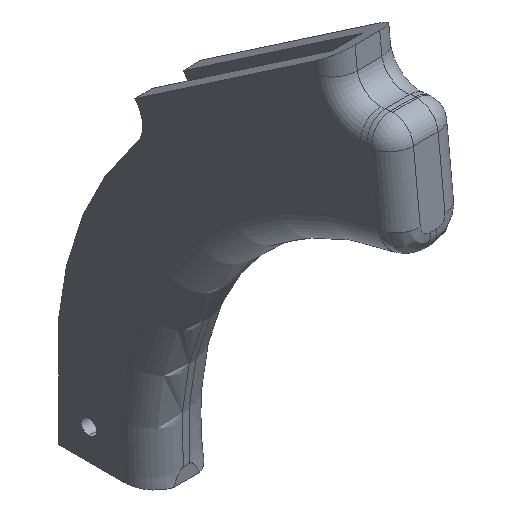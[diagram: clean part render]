
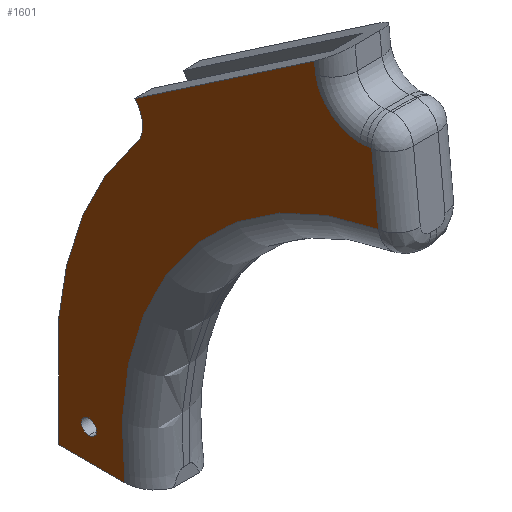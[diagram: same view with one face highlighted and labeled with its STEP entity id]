
A CAD part, isometric view. The second image highlights one B-rep face of the part: STEP entity #1601.
In plain terms, the highlighted planar face has unit normal (-1, 0, 0).
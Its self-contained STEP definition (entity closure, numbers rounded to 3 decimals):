
#111 = ORIENTED_EDGE ( 'NONE', *, *, #1581, .F. ) ;
#112 = ORIENTED_EDGE ( 'NONE', *, *, #1582, .T. ) ;
#113 = ORIENTED_EDGE ( 'NONE', *, *, #1477, .F. ) ;
#114 = ORIENTED_EDGE ( 'NONE', *, *, #1539, .T. ) ;
#117 = ORIENTED_EDGE ( 'NONE', *, *, #1546, .F. ) ;
#118 = ORIENTED_EDGE ( 'NONE', *, *, #1476, .F. ) ;
#121 = ORIENTED_EDGE ( 'NONE', *, *, #1494, .T. ) ;
#122 = ORIENTED_EDGE ( 'NONE', *, *, #1587, .T. ) ;
#123 = ORIENTED_EDGE ( 'NONE', *, *, #1571, .T. ) ;
#127 = ORIENTED_EDGE ( 'NONE', *, *, #1590, .F. ) ;
#128 = ORIENTED_EDGE ( 'NONE', *, *, #1574, .T. ) ;
#129 = ORIENTED_EDGE ( 'NONE', *, *, #1576, .F. ) ;
#130 = ORIENTED_EDGE ( 'NONE', *, *, #1589, .T. ) ;
#136 = EDGE_LOOP ( 'NONE', ( #127, #113 ) ) ;
#155 = EDGE_LOOP ( 'NONE', ( #121, #112, #130, #118, #114, #117, #129, #111, #128, #123, #122 ) ) ;
#310 = CARTESIAN_POINT ( 'NONE',  ( -11.112, -83.313, 10.48 ) ) ;
#319 = DIRECTION ( 'NONE',  ( 0., 0., 1. ) ) ;
#320 = CARTESIAN_POINT ( 'NONE',  ( -11.112, 12.933, 89.824 ) ) ;
#321 = DIRECTION ( 'NONE',  ( 1., 0., 0. ) ) ;
#338 = DIRECTION ( 'NONE',  ( 1., 0., 0. ) ) ;
#340 = DIRECTION ( 'NONE',  ( 0., 0., 1. ) ) ;
#440 = LINE ( 'NONE', #441, #1780 ) ;
#441 = CARTESIAN_POINT ( 'NONE',  ( -11.112, -72.744, 125.05 ) ) ;
#466 = DIRECTION ( 'NONE',  ( 0., 0., -1. ) ) ;
#467 = CARTESIAN_POINT ( 'NONE',  ( -11.112, 31.75, 19.685 ) ) ;
#468 = CARTESIAN_POINT ( 'NONE',  ( -11.112, -92.94, -2.565 ) ) ;
#473 = LINE ( 'NONE', #474, #1796 ) ;
#474 = CARTESIAN_POINT ( 'NONE',  ( -11.112, 24.13, -16.51 ) ) ;
#476 = DIRECTION ( 'NONE',  ( 0., 0.101, 0.995 ) ) ;
#477 = DIRECTION ( 'NONE',  ( 1., 0., 0. ) ) ;
#479 = DIRECTION ( 'NONE',  ( 0., 0., 1. ) ) ;
#483 = LINE ( 'NONE', #467, #1795 ) ;
#490 = CARTESIAN_POINT ( 'NONE',  ( -11.112, -69.095, 136.361 ) ) ;
#491 = DIRECTION ( 'NONE',  ( 1., 0., 0. ) ) ;
#498 = CARTESIAN_POINT ( 'NONE',  ( -11.112, -77.504, 122.176 ) ) ;
#499 = LINE ( 'NONE', #513, #1824 ) ;
#502 = DIRECTION ( 'NONE',  ( 0., 0., 1. ) ) ;
#505 = DIRECTION ( 'NONE',  ( 0., 0., -1. ) ) ;
#506 = CARTESIAN_POINT ( 'NONE',  ( -11.113, 21.59, -6.35 ) ) ;
#507 = DIRECTION ( 'NONE',  ( -1., 0., 0. ) ) ;
#512 = DIRECTION ( 'NONE',  ( 0., 0.995, -0.101 ) ) ;
#513 = CARTESIAN_POINT ( 'NONE',  ( -11.112, -53.555, 141.256 ) ) ;
#514 = LINE ( 'NONE', #498, #1812 ) ;
#516 = DIRECTION ( 'NONE',  ( 0., 0.101, 0.995 ) ) ;
#520 = DIRECTION ( 'NONE',  ( 0., 1., 0. ) ) ;
#527 = PLANE ( 'NONE',  #1810 ) ;
#559 = CARTESIAN_POINT ( 'NONE',  ( -11.112, 0., 0. ) ) ;
#566 = DIRECTION ( 'NONE',  ( 1., 0., 0. ) ) ;
#574 = DIRECTION ( 'NONE',  ( 0., 0., -1. ) ) ;
#996 = VERTEX_POINT ( 'NONE', #1107 ) ;
#998 = VERTEX_POINT ( 'NONE', #1091 ) ;
#1009 = VERTEX_POINT ( 'NONE', #1085 ) ;
#1014 = VERTEX_POINT ( 'NONE', #1086 ) ;
#1015 = VERTEX_POINT ( 'NONE', #1100 ) ;
#1022 = VERTEX_POINT ( 'NONE', #1136 ) ;
#1023 = VERTEX_POINT ( 'NONE', #1119 ) ;
#1032 = VERTEX_POINT ( 'NONE', #1134 ) ;
#1034 = VERTEX_POINT ( 'NONE', #1140 ) ;
#1043 = VERTEX_POINT ( 'NONE', #1129 ) ;
#1045 = VERTEX_POINT ( 'NONE', #1135 ) ;
#1046 = VERTEX_POINT ( 'NONE', #1141 ) ;
#1049 = VERTEX_POINT ( 'NONE', #1111 ) ;
#1085 = CARTESIAN_POINT ( 'NONE',  ( -11.113, -69.095, 121.361 ) ) ;
#1086 = CARTESIAN_POINT ( 'NONE',  ( -11.112, 31.75, -16.51 ) ) ;
#1091 = CARTESIAN_POINT ( 'NONE',  ( -11.112, -71.647, 121.58 ) ) ;
#1100 = CARTESIAN_POINT ( 'NONE',  ( -11.112, -54.314, 133.809 ) ) ;
#1107 = CARTESIAN_POINT ( 'NONE',  ( -11.112, 6.321, 83.212 ) ) ;
#1111 = CARTESIAN_POINT ( 'NONE',  ( -11.112, -53.939, 137.484 ) ) ;
#1119 = CARTESIAN_POINT ( 'NONE',  ( -11.113, 21.59, -3.81 ) ) ;
#1129 = CARTESIAN_POINT ( 'NONE',  ( -11.112, 31.75, 19.685 ) ) ;
#1134 = CARTESIAN_POINT ( 'NONE',  ( -11.112, 6.321, 96.436 ) ) ;
#1135 = CARTESIAN_POINT ( 'NONE',  ( -11.112, 9.553, -16.51 ) ) ;
#1136 = CARTESIAN_POINT ( 'NONE',  ( -11.113, 21.59, -8.89 ) ) ;
#1140 = CARTESIAN_POINT ( 'NONE',  ( -11.112, -75.361, 99.367 ) ) ;
#1141 = CARTESIAN_POINT ( 'NONE',  ( -11.112, -73.082, 121.726 ) ) ;
#1159 = CARTESIAN_POINT ( 'NONE',  ( -11.113, 21.59, -6.35 ) ) ;
#1175 = DIRECTION ( 'NONE',  ( 0., -0.826, 0.563 ) ) ;
#1182 = CARTESIAN_POINT ( 'NONE',  ( -11.112, 46.873, 68.813 ) ) ;
#1183 = LINE ( 'NONE', #1182, #1700 ) ;
#1193 = DIRECTION ( 'NONE',  ( -1., 0., 0. ) ) ;
#1195 = DIRECTION ( 'NONE',  ( 0., 0., 1. ) ) ;
#1232 = CARTESIAN_POINT ( 'NONE',  ( -11.112, -69.095, 136.361 ) ) ;
#1240 = DIRECTION ( 'NONE',  ( 0., 0., -1. ) ) ;
#1255 = DIRECTION ( 'NONE',  ( 1., 0., 0. ) ) ;
#1443 = CIRCLE ( 'NONE', #1791, 15. ) ;
#1446 = CIRCLE ( 'NONE', #1825, 2.54 ) ;
#1463 = CIRCLE ( 'NONE', #1773, 103.437 ) ;
#1476 = EDGE_CURVE ( 'NONE', #1032, #1049, #1183, .T. ) ;
#1477 = EDGE_CURVE ( 'NONE', #1022, #1023, #1644, .T. ) ;
#1494 = EDGE_CURVE ( 'NONE', #998, #1009, #1639, .T. ) ;
#1539 = EDGE_CURVE ( 'NONE', #1032, #996, #1671, .T. ) ;
#1546 = EDGE_CURVE ( 'NONE', #1043, #996, #1665, .T. ) ;
#1571 = EDGE_CURVE ( 'NONE', #1034, #1046, #440, .T. ) ;
#1574 = EDGE_CURVE ( 'NONE', #1045, #1034, #1463, .T. ) ;
#1576 = EDGE_CURVE ( 'NONE', #1014, #1043, #483, .T. ) ;
#1581 = EDGE_CURVE ( 'NONE', #1045, #1014, #473, .T. ) ;
#1582 = EDGE_CURVE ( 'NONE', #1009, #1015, #1443, .T. ) ;
#1587 = EDGE_CURVE ( 'NONE', #1046, #998, #514, .T. ) ;
#1589 = EDGE_CURVE ( 'NONE', #1015, #1049, #499, .T. ) ;
#1590 = EDGE_CURVE ( 'NONE', #1023, #1022, #1446, .T. ) ;
#1601 = ADVANCED_FACE ( 'NONE', ( #1829, #1821 ), #527, .F. ) ;
#1639 = CIRCLE ( 'NONE', #1708, 15. ) ;
#1644 = CIRCLE ( 'NONE', #1692, 2.54 ) ;
#1665 = CIRCLE ( 'NONE', #1746, 115.431 ) ;
#1671 = CIRCLE ( 'NONE', #1737, 9.351 ) ;
#1692 = AXIS2_PLACEMENT_3D ( 'NONE', #1159, #1193, #1195 ) ;
#1700 = VECTOR ( 'NONE', #1175, 1000. ) ;
#1708 = AXIS2_PLACEMENT_3D ( 'NONE', #1232, #1255, #1240 ) ;
#1737 = AXIS2_PLACEMENT_3D ( 'NONE', #320, #321, #319 ) ;
#1746 = AXIS2_PLACEMENT_3D ( 'NONE', #310, #338, #340 ) ;
#1773 = AXIS2_PLACEMENT_3D ( 'NONE', #468, #477, #466 ) ;
#1780 = VECTOR ( 'NONE', #476, 1000. ) ;
#1791 = AXIS2_PLACEMENT_3D ( 'NONE', #490, #491, #505 ) ;
#1795 = VECTOR ( 'NONE', #479, 1000. ) ;
#1796 = VECTOR ( 'NONE', #520, 1000. ) ;
#1810 = AXIS2_PLACEMENT_3D ( 'NONE', #559, #566, #574 ) ;
#1812 = VECTOR ( 'NONE', #512, 1000. ) ;
#1821 = FACE_BOUND ( 'NONE', #136, .T. ) ;
#1824 = VECTOR ( 'NONE', #516, 1000. ) ;
#1825 = AXIS2_PLACEMENT_3D ( 'NONE', #506, #507, #502 ) ;
#1829 = FACE_OUTER_BOUND ( 'NONE', #155, .T. ) ;
